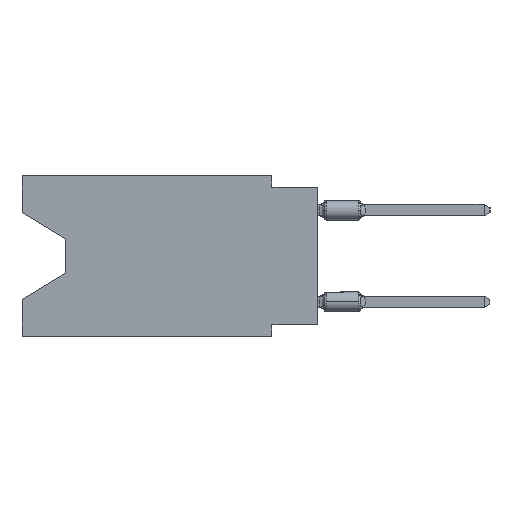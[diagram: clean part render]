
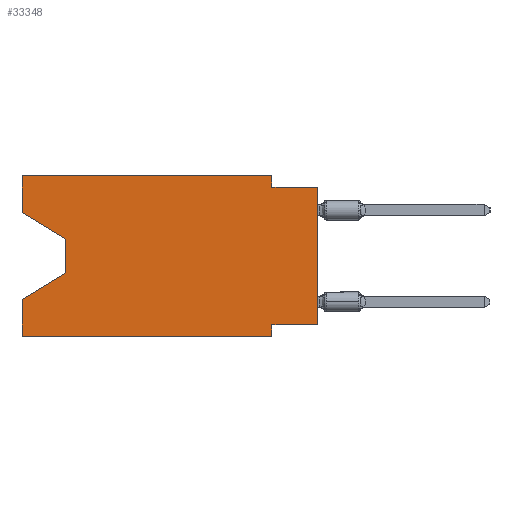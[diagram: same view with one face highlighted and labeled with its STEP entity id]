
A CAD part, left-side view. The second image highlights one B-rep face of the part: STEP entity #33348.
In plain terms, the highlighted planar face has unit normal (-1, 0, 0).
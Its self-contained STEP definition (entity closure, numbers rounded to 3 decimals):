
#1184 = ORIENTED_EDGE ( 'NONE', *, *, #6167, .T. ) ;
#2079 = VECTOR ( 'NONE', #16150, 1000. ) ;
#2933 = LINE ( 'NONE', #37653, #39162 ) ;
#3264 = DIRECTION ( 'NONE',  ( 1., 0., 0. ) ) ;
#3595 = VERTEX_POINT ( 'NONE', #15470 ) ;
#4310 = CARTESIAN_POINT ( 'NONE',  ( 0., 16.383, 0. ) ) ;
#5846 = DIRECTION ( 'NONE',  ( 0., 0., 1. ) ) ;
#6167 = EDGE_CURVE ( 'NONE', #3595, #54269, #27139, .T. ) ;
#6528 = LINE ( 'NONE', #33790, #33647 ) ;
#7573 = CARTESIAN_POINT ( 'NONE',  ( 0., 16.383, 0. ) ) ;
#7998 = LINE ( 'NONE', #4310, #16325 ) ;
#8099 = DIRECTION ( 'NONE',  ( 0., 0., -1. ) ) ;
#8231 = CARTESIAN_POINT ( 'NONE',  ( 0., 2.54, -0.635 ) ) ;
#8667 = VECTOR ( 'NONE', #41401, 1000. ) ;
#10297 = VECTOR ( 'NONE', #10733, 1000. ) ;
#10701 = CARTESIAN_POINT ( 'NONE',  ( 0., 16.383, -2.038 ) ) ;
#10733 = DIRECTION ( 'NONE',  ( 0., 0., -1. ) ) ;
#10930 = CARTESIAN_POINT ( 'NONE',  ( 0., 2.54, -8.89 ) ) ;
#12383 = CARTESIAN_POINT ( 'NONE',  ( 0., 16.383, 0. ) ) ;
#13105 = CARTESIAN_POINT ( 'NONE',  ( 0., 16.383, -6.852 ) ) ;
#13256 = CARTESIAN_POINT ( 'NONE',  ( 0., 13.97, -5.385 ) ) ;
#13542 = EDGE_CURVE ( 'NONE', #44247, #54269, #6528, .T. ) ;
#14032 = EDGE_CURVE ( 'NONE', #21827, #27511, #2933, .T. ) ;
#15277 = LINE ( 'NONE', #45182, #10297 ) ;
#15470 = CARTESIAN_POINT ( 'NONE',  ( 0., 0., -8.255 ) ) ;
#15474 = LINE ( 'NONE', #10930, #45431 ) ;
#16150 = DIRECTION ( 'NONE',  ( 0., 0., -1. ) ) ;
#16325 = VECTOR ( 'NONE', #55263, 1000. ) ;
#16503 = EDGE_CURVE ( 'NONE', #53887, #21827, #20434, .T. ) ;
#16711 = ORIENTED_EDGE ( 'NONE', *, *, #13542, .F. ) ;
#18037 = EDGE_LOOP ( 'NONE', ( #28632, #45208, #21553, #30690, #45260, #44627, #35543, #1184, #16711, #33605, #39707, #50845 ) ) ;
#18638 = VERTEX_POINT ( 'NONE', #23582 ) ;
#20434 = LINE ( 'NONE', #33235, #2079 ) ;
#21011 = VECTOR ( 'NONE', #40704, 1000. ) ;
#21553 = ORIENTED_EDGE ( 'NONE', *, *, #14032, .T. ) ;
#21827 = VERTEX_POINT ( 'NONE', #13256 ) ;
#23195 = DIRECTION ( 'NONE',  ( 0., 0., -1. ) ) ;
#23243 = DIRECTION ( 'NONE',  ( 0., -0.855, -0.519 ) ) ;
#23368 = LINE ( 'NONE', #49554, #21011 ) ;
#23582 = CARTESIAN_POINT ( 'NONE',  ( 0., 16.383, -2.038 ) ) ;
#23761 = CARTESIAN_POINT ( 'NONE',  ( 0., 13.97, -3.505 ) ) ;
#24089 = CARTESIAN_POINT ( 'NONE',  ( 0., 16.383, -8.89 ) ) ;
#26914 = EDGE_CURVE ( 'NONE', #3595, #45072, #28303, .T. ) ;
#27139 = LINE ( 'NONE', #35378, #30522 ) ;
#27511 = VERTEX_POINT ( 'NONE', #13105 ) ;
#27753 = LINE ( 'NONE', #48815, #32136 ) ;
#28303 = LINE ( 'NONE', #49095, #8667 ) ;
#28342 = LINE ( 'NONE', #10701, #41914 ) ;
#28632 = ORIENTED_EDGE ( 'NONE', *, *, #29030, .T. ) ;
#28682 = VERTEX_POINT ( 'NONE', #54193 ) ;
#28919 = CARTESIAN_POINT ( 'NONE',  ( 0., 2.54, -8.255 ) ) ;
#29030 = EDGE_CURVE ( 'NONE', #18638, #53887, #28342, .T. ) ;
#30140 = EDGE_CURVE ( 'NONE', #45072, #28682, #15474, .T. ) ;
#30522 = VECTOR ( 'NONE', #35102, 1000. ) ;
#30690 = ORIENTED_EDGE ( 'NONE', *, *, #38538, .F. ) ;
#31286 = VECTOR ( 'NONE', #53789, 1000. ) ;
#32136 = VECTOR ( 'NONE', #5846, 1000. ) ;
#33163 = PLANE ( 'NONE',  #33852 ) ;
#33235 = CARTESIAN_POINT ( 'NONE',  ( 0., 13.97, -3.505 ) ) ;
#33348 = ADVANCED_FACE ( 'NONE', ( #47103 ), #33163, .F. ) ;
#33605 = ORIENTED_EDGE ( 'NONE', *, *, #38144, .F. ) ;
#33647 = VECTOR ( 'NONE', #51184, 1000. ) ;
#33790 = CARTESIAN_POINT ( 'NONE',  ( 0., 0., -0.635 ) ) ;
#33852 = AXIS2_PLACEMENT_3D ( 'NONE', #12383, #3264, #8099 ) ;
#35095 = CARTESIAN_POINT ( 'NONE',  ( 0., 2.54, 0. ) ) ;
#35102 = DIRECTION ( 'NONE',  ( 0., 0., 1. ) ) ;
#35378 = CARTESIAN_POINT ( 'NONE',  ( 0., 0., 0. ) ) ;
#35470 = VERTEX_POINT ( 'NONE', #35095 ) ;
#35543 = ORIENTED_EDGE ( 'NONE', *, *, #26914, .F. ) ;
#36406 = CARTESIAN_POINT ( 'NONE',  ( 0., 16.383, 0. ) ) ;
#37653 = CARTESIAN_POINT ( 'NONE',  ( 0., 13.97, -5.385 ) ) ;
#37768 = EDGE_CURVE ( 'NONE', #44995, #35470, #40970, .T. ) ;
#38144 = EDGE_CURVE ( 'NONE', #35470, #44247, #15277, .T. ) ;
#38538 = EDGE_CURVE ( 'NONE', #40848, #27511, #27753, .T. ) ;
#39162 = VECTOR ( 'NONE', #42775, 1000. ) ;
#39707 = ORIENTED_EDGE ( 'NONE', *, *, #37768, .F. ) ;
#40704 = DIRECTION ( 'NONE',  ( 0., -1., 0. ) ) ;
#40848 = VERTEX_POINT ( 'NONE', #24089 ) ;
#40970 = LINE ( 'NONE', #36406, #31286 ) ;
#41321 = EDGE_CURVE ( 'NONE', #40848, #28682, #23368, .T. ) ;
#41401 = DIRECTION ( 'NONE',  ( 0., 1., 0. ) ) ;
#41914 = VECTOR ( 'NONE', #23243, 1000. ) ;
#42775 = DIRECTION ( 'NONE',  ( 0., 0.855, -0.519 ) ) ;
#42945 = EDGE_CURVE ( 'NONE', #18638, #44995, #7998, .T. ) ;
#43644 = CARTESIAN_POINT ( 'NONE',  ( 0., 0., -0.635 ) ) ;
#44247 = VERTEX_POINT ( 'NONE', #8231 ) ;
#44627 = ORIENTED_EDGE ( 'NONE', *, *, #30140, .F. ) ;
#44995 = VERTEX_POINT ( 'NONE', #7573 ) ;
#45072 = VERTEX_POINT ( 'NONE', #28919 ) ;
#45182 = CARTESIAN_POINT ( 'NONE',  ( 0., 2.54, 0. ) ) ;
#45208 = ORIENTED_EDGE ( 'NONE', *, *, #16503, .T. ) ;
#45260 = ORIENTED_EDGE ( 'NONE', *, *, #41321, .T. ) ;
#45431 = VECTOR ( 'NONE', #23195, 1000. ) ;
#47103 = FACE_OUTER_BOUND ( 'NONE', #18037, .T. ) ;
#48815 = CARTESIAN_POINT ( 'NONE',  ( 0., 16.383, 0. ) ) ;
#49095 = CARTESIAN_POINT ( 'NONE',  ( 0., 0., -8.255 ) ) ;
#49554 = CARTESIAN_POINT ( 'NONE',  ( 0., 16.383, -8.89 ) ) ;
#50845 = ORIENTED_EDGE ( 'NONE', *, *, #42945, .F. ) ;
#51184 = DIRECTION ( 'NONE',  ( 0., -1., 0. ) ) ;
#53789 = DIRECTION ( 'NONE',  ( 0., -1., 0. ) ) ;
#53887 = VERTEX_POINT ( 'NONE', #23761 ) ;
#54193 = CARTESIAN_POINT ( 'NONE',  ( 0., 2.54, -8.89 ) ) ;
#54269 = VERTEX_POINT ( 'NONE', #43644 ) ;
#55263 = DIRECTION ( 'NONE',  ( 0., 0., 1. ) ) ;
